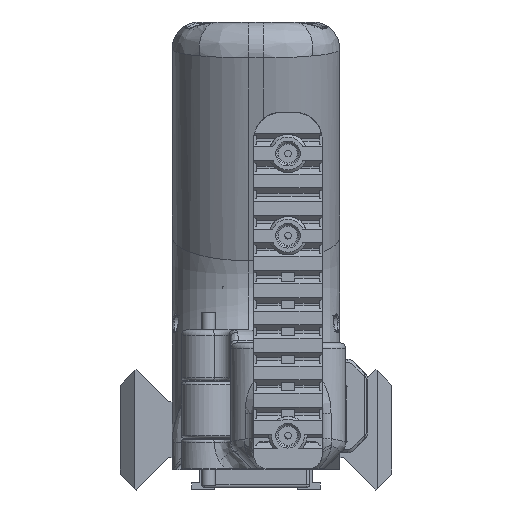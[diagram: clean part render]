
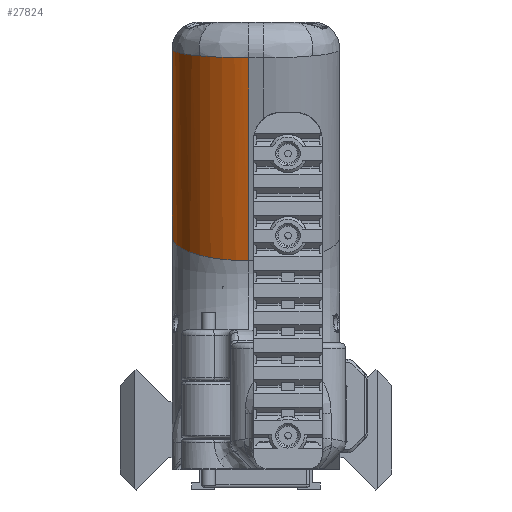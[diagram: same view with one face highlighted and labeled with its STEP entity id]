
A CAD part, left-side view. The second image highlights one B-rep face of the part: STEP entity #27824.
In plain terms, the highlighted cylindrical face has radius 14 mm (diameter 28 mm), a partial arc.
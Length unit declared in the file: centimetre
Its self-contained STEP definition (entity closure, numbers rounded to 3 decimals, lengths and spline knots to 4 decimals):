
#757=ELLIPSE($,#30378,1.4302,1.4);
#758=ELLIPSE($,#30379,1.4302,1.4);
#2595=LINE($,#45385,#4769);
#2841=LINE($,#48354,#5015);
#4769=VECTOR($,#35007,3.6015);
#5015=VECTOR($,#35955,3.894);
#7688=FACE_OUTER_BOUND($,#9501,.T.);
#9501=EDGE_LOOP($,(#23689,#23690,#23691,#23692,#23693));
#10828=CIRCLE($,#30377,1.4);
#12474=VERTEX_POINT($,#45382);
#12475=VERTEX_POINT($,#45384);
#12888=VERTEX_POINT($,#48352);
#12889=VERTEX_POINT($,#48353);
#13293=VERTEX_POINT($,#51597);
#15726=EDGE_CURVE($,#12475,#12474,#2595,.T.);
#16317=EDGE_CURVE($,#12888,#12889,#2841,.T.);
#16939=EDGE_CURVE($,#12888,#12474,#10828,.T.);
#16940=EDGE_CURVE($,#13293,#12889,#757,.T.);
#16941=EDGE_CURVE($,#12475,#13293,#758,.T.);
#23689=ORIENTED_EDGE($,*,*,#15726,.T.);
#23690=ORIENTED_EDGE($,*,*,#16939,.F.);
#23691=ORIENTED_EDGE($,*,*,#16317,.T.);
#23692=ORIENTED_EDGE($,*,*,#16940,.F.);
#23693=ORIENTED_EDGE($,*,*,#16941,.F.);
#26487=CYLINDRICAL_SURFACE($,#30376,1.4);
#27824=ADVANCED_FACE($,(#7688),#26487,.T.);
#30376=AXIS2_PLACEMENT_3D($,#51595,#37011,#37012);
#30377=AXIS2_PLACEMENT_3D($,#51596,#37013,#37014);
#30378=AXIS2_PLACEMENT_3D($,#51598,#37015,#37016);
#30379=AXIS2_PLACEMENT_3D($,#51599,#37017,#37018);
#35007=DIRECTION($,(0.309,0.,-0.951));
#35955=DIRECTION($,(-0.309,0.,0.951));
#37011=DIRECTION('center_axis',(-0.309,0.,0.951));
#37012=DIRECTION('ref_axis',(-0.672,0.707,-0.219));
#37013=DIRECTION('center_axis',(0.309,0.,-0.951));
#37014=DIRECTION('ref_axis',(-0.951,0.,-0.309));
#37015=DIRECTION('center_axis',(-0.108,0.,
0.994));
#37016=DIRECTION('ref_axis',(-0.994,0.,-0.108));
#37017=DIRECTION('center_axis',(-0.108,0.,
0.994));
#37018=DIRECTION('ref_axis',(0.994,0.,0.108));
#45382=CARTESIAN_POINT('',(-5.5323,11.505,0.241));
#45384=CARTESIAN_POINT('',(-6.6452,11.505,3.6662));
#45385=CARTESIAN_POINT($,(-5.8254,11.505,1.1431));
#48352=CARTESIAN_POINT('',(-6.8637,10.105,-0.1917));
#48353=CARTESIAN_POINT('',(-8.067,10.105,3.5117));
#48354=CARTESIAN_POINT($,(-6.786,10.105,-0.4308));
#51595=CARTESIAN_POINT('Origin',(-5.8254,10.105,1.1431));
#51596=CARTESIAN_POINT('Origin',(-5.5323,10.105,0.241));
#51597=CARTESIAN_POINT('',(-7.7351,11.004,3.5478));
#51598=CARTESIAN_POINT('Origin',(-6.6452,10.105,3.6662));
#51599=CARTESIAN_POINT('Origin',(-6.6452,10.105,3.6662));
